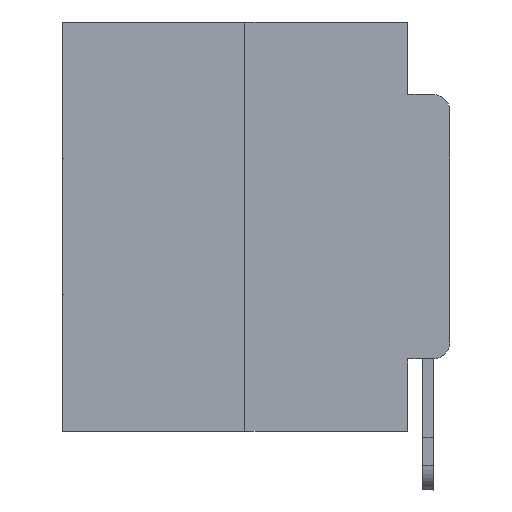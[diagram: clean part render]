
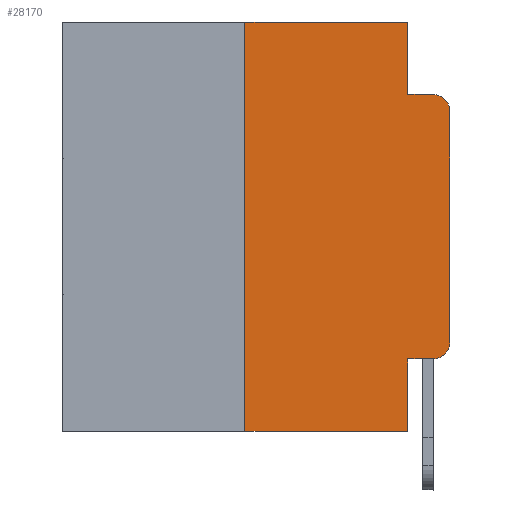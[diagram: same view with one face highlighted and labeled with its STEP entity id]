
A CAD part, left-side view. The second image highlights one B-rep face of the part: STEP entity #28170.
In plain terms, the highlighted planar face has unit normal (-1, 0, 0).
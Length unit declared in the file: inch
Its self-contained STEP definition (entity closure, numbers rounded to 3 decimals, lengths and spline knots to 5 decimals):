
#36 = AXIS2_PLACEMENT_3D ( 'NONE', #8224, #28584, #23990 ) ;
#792 = ORIENTED_EDGE ( 'NONE', *, *, #2212, .F. ) ;
#1708 = DIRECTION ( 'NONE',  ( 0., 0., -1. ) ) ;
#1855 = ORIENTED_EDGE ( 'NONE', *, *, #16645, .F. ) ;
#2212 = EDGE_CURVE ( 'NONE', #21345, #11055, #28645, .T. ) ;
#2528 = CARTESIAN_POINT ( 'NONE',  ( 0., 0.051, -0.4115 ) ) ;
#2829 = DIRECTION ( 'NONE',  ( 0., -1., 0. ) ) ;
#3201 = VECTOR ( 'NONE', #11727, 39.37008 ) ;
#3476 = CARTESIAN_POINT ( 'NONE',  ( 0., 0.473, 0. ) ) ;
#3524 = VECTOR ( 'NONE', #15299, 39.37008 ) ;
#3611 = CIRCLE ( 'NONE', #17401, 0.02 ) ;
#4277 = CIRCLE ( 'NONE', #36, 0.02 ) ;
#4423 = ORIENTED_EDGE ( 'NONE', *, *, #27594, .F. ) ;
#4729 = ORIENTED_EDGE ( 'NONE', *, *, #23625, .T. ) ;
#5069 = VERTEX_POINT ( 'NONE', #6980 ) ;
#5205 = CARTESIAN_POINT ( 'NONE',  ( 0., 0., -0.1085 ) ) ;
#6229 = ORIENTED_EDGE ( 'NONE', *, *, #20766, .F. ) ;
#6548 = VERTEX_POINT ( 'NONE', #12585 ) ;
#6980 = CARTESIAN_POINT ( 'NONE',  ( 0., 0.051, 0. ) ) ;
#7550 = LINE ( 'NONE', #7691, #20832 ) ;
#7691 = CARTESIAN_POINT ( 'NONE',  ( 0., 0.473, 0. ) ) ;
#7853 = VERTEX_POINT ( 'NONE', #5205 ) ;
#8224 = CARTESIAN_POINT ( 'NONE',  ( 0., 0.02, -0.1085 ) ) ;
#8288 = CARTESIAN_POINT ( 'NONE',  ( 0., 0.051, -0.0885 ) ) ;
#8611 = VERTEX_POINT ( 'NONE', #11492 ) ;
#8672 = LINE ( 'NONE', #13152, #22051 ) ;
#9423 = EDGE_CURVE ( 'NONE', #5069, #21345, #23165, .T. ) ;
#10440 = CARTESIAN_POINT ( 'NONE',  ( 0., 0.051, -0.4115 ) ) ;
#10768 = CARTESIAN_POINT ( 'NONE',  ( 0., 0.25, -0.5 ) ) ;
#10935 = VERTEX_POINT ( 'NONE', #10768 ) ;
#11055 = VERTEX_POINT ( 'NONE', #27373 ) ;
#11372 = ORIENTED_EDGE ( 'NONE', *, *, #27034, .T. ) ;
#11492 = CARTESIAN_POINT ( 'NONE',  ( 0., 0.02, -0.4115 ) ) ;
#11692 = EDGE_CURVE ( 'NONE', #6548, #7853, #19452, .T. ) ;
#11727 = DIRECTION ( 'NONE',  ( 0., 0., -1. ) ) ;
#12552 = DIRECTION ( 'NONE',  ( 1., 0., 0. ) ) ;
#12585 = CARTESIAN_POINT ( 'NONE',  ( 0., 0., -0.3915 ) ) ;
#12965 = VECTOR ( 'NONE', #22550, 39.37008 ) ;
#13152 = CARTESIAN_POINT ( 'NONE',  ( 0., 0.051, 0. ) ) ;
#13535 = LINE ( 'NONE', #2528, #16054 ) ;
#13641 = ORIENTED_EDGE ( 'NONE', *, *, #25902, .T. ) ;
#13844 = EDGE_CURVE ( 'NONE', #7853, #11055, #4277, .T. ) ;
#14796 = FACE_OUTER_BOUND ( 'NONE', #26693, .T. ) ;
#15146 = LINE ( 'NONE', #24501, #12965 ) ;
#15299 = DIRECTION ( 'NONE',  ( 0., -1., 0. ) ) ;
#15387 = ORIENTED_EDGE ( 'NONE', *, *, #13844, .T. ) ;
#15612 = CARTESIAN_POINT ( 'NONE',  ( 0., 0.051, -0.5 ) ) ;
#16054 = VECTOR ( 'NONE', #2829, 39.37008 ) ;
#16508 = DIRECTION ( 'NONE',  ( -1., 0., 0. ) ) ;
#16587 = CARTESIAN_POINT ( 'NONE',  ( 0., 0.473, -0.5 ) ) ;
#16638 = DIRECTION ( 'NONE',  ( 0., -1., 0. ) ) ;
#16645 = EDGE_CURVE ( 'NONE', #10935, #19563, #15146, .T. ) ;
#17401 = AXIS2_PLACEMENT_3D ( 'NONE', #20794, #16508, #25567 ) ;
#18530 = VERTEX_POINT ( 'NONE', #15612 ) ;
#18774 = CARTESIAN_POINT ( 'NONE',  ( 0., 0.25, 0. ) ) ;
#19074 = LINE ( 'NONE', #16587, #26031 ) ;
#19303 = DIRECTION ( 'NONE',  ( 0., 0., 1. ) ) ;
#19434 = VECTOR ( 'NONE', #19303, 39.37008 ) ;
#19452 = LINE ( 'NONE', #23335, #19434 ) ;
#19563 = VERTEX_POINT ( 'NONE', #18774 ) ;
#20384 = CARTESIAN_POINT ( 'NONE',  ( 0., 0.051, -0.0885 ) ) ;
#20766 = EDGE_CURVE ( 'NONE', #21005, #18530, #8672, .T. ) ;
#20777 = CARTESIAN_POINT ( 'NONE',  ( 0., 0.051, 0. ) ) ;
#20794 = CARTESIAN_POINT ( 'NONE',  ( 0., 0.02, -0.3915 ) ) ;
#20832 = VECTOR ( 'NONE', #16638, 39.37008 ) ;
#21005 = VERTEX_POINT ( 'NONE', #10440 ) ;
#21345 = VERTEX_POINT ( 'NONE', #20384 ) ;
#21605 = DIRECTION ( 'NONE',  ( 0., 0., -1. ) ) ;
#22051 = VECTOR ( 'NONE', #1708, 39.37008 ) ;
#22550 = DIRECTION ( 'NONE',  ( 0., 0., 1. ) ) ;
#23165 = LINE ( 'NONE', #20777, #3201 ) ;
#23335 = CARTESIAN_POINT ( 'NONE',  ( 0., 0., 0. ) ) ;
#23625 = EDGE_CURVE ( 'NONE', #8611, #6548, #3611, .T. ) ;
#23840 = PLANE ( 'NONE',  #26073 ) ;
#23990 = DIRECTION ( 'NONE',  ( 0., 0., -1. ) ) ;
#24501 = CARTESIAN_POINT ( 'NONE',  ( 0., 0.25, 0. ) ) ;
#24771 = ORIENTED_EDGE ( 'NONE', *, *, #11692, .T. ) ;
#25567 = DIRECTION ( 'NONE',  ( 0., 0., -1. ) ) ;
#25649 = DIRECTION ( 'NONE',  ( 0., -1., 0. ) ) ;
#25902 = EDGE_CURVE ( 'NONE', #10935, #18530, #19074, .T. ) ;
#26031 = VECTOR ( 'NONE', #25649, 39.37008 ) ;
#26073 = AXIS2_PLACEMENT_3D ( 'NONE', #3476, #12552, #21605 ) ;
#26646 = ORIENTED_EDGE ( 'NONE', *, *, #9423, .F. ) ;
#26693 = EDGE_LOOP ( 'NONE', ( #24771, #15387, #792, #26646, #4423, #1855, #13641, #6229, #11372, #4729 ) ) ;
#27034 = EDGE_CURVE ( 'NONE', #21005, #8611, #13535, .T. ) ;
#27373 = CARTESIAN_POINT ( 'NONE',  ( 0., 0.02, -0.0885 ) ) ;
#27594 = EDGE_CURVE ( 'NONE', #19563, #5069, #7550, .T. ) ;
#28170 = ADVANCED_FACE ( 'NONE', ( #14796 ), #23840, .F. ) ;
#28584 = DIRECTION ( 'NONE',  ( -1., 0., 0. ) ) ;
#28645 = LINE ( 'NONE', #8288, #3524 ) ;
